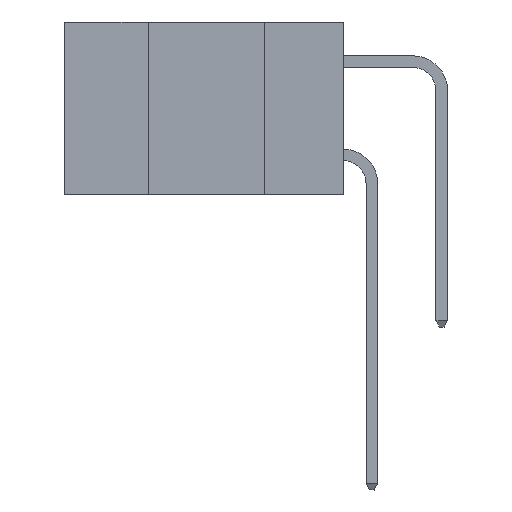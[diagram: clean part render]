
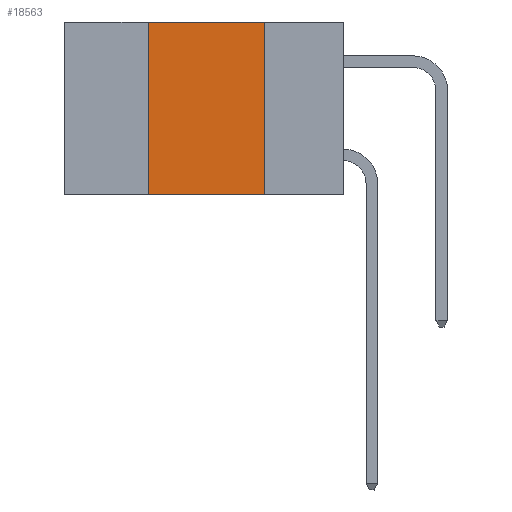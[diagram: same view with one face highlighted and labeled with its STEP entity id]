
A CAD part, left-side view. The second image highlights one B-rep face of the part: STEP entity #18563.
In plain terms, the highlighted planar face has unit normal (-1, 0, 0).
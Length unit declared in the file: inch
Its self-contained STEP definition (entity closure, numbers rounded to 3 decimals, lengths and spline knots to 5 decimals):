
#538 = CARTESIAN_POINT ( 'NONE',  ( 0., 0.42, -0.37 ) ) ;
#1553 = CARTESIAN_POINT ( 'NONE',  ( 0., 0.6, 0. ) ) ;
#1565 = VECTOR ( 'NONE', #15667, 39.37008 ) ;
#1734 = CARTESIAN_POINT ( 'NONE',  ( 0., 0.42, 0. ) ) ;
#2857 = EDGE_CURVE ( 'NONE', #12236, #12527, #21945, .T. ) ;
#3098 = PLANE ( 'NONE',  #3495 ) ;
#3495 = AXIS2_PLACEMENT_3D ( 'NONE', #11609, #20102, #5338 ) ;
#4161 = EDGE_CURVE ( 'NONE', #12236, #16341, #20436, .T. ) ;
#5338 = DIRECTION ( 'NONE',  ( 0., 0., -1. ) ) ;
#5817 = CARTESIAN_POINT ( 'NONE',  ( 0., 0.17, 0. ) ) ;
#6176 = VECTOR ( 'NONE', #16525, 39.37008 ) ;
#9912 = VERTEX_POINT ( 'NONE', #5817 ) ;
#11609 = CARTESIAN_POINT ( 'NONE',  ( 0., 0.6, 0. ) ) ;
#11755 = EDGE_LOOP ( 'NONE', ( #21059, #25407, #21462, #27111 ) ) ;
#12236 = VERTEX_POINT ( 'NONE', #538 ) ;
#12527 = VERTEX_POINT ( 'NONE', #23983 ) ;
#13703 = FACE_OUTER_BOUND ( 'NONE', #11755, .T. ) ;
#15221 = VECTOR ( 'NONE', #20825, 39.37008 ) ;
#15667 = DIRECTION ( 'NONE',  ( 0., -1., 0. ) ) ;
#16341 = VERTEX_POINT ( 'NONE', #1734 ) ;
#16525 = DIRECTION ( 'NONE',  ( 0., 0., 1. ) ) ;
#18563 = ADVANCED_FACE ( 'NONE', ( #13703 ), #3098, .F. ) ;
#19992 = CARTESIAN_POINT ( 'NONE',  ( 0., 0.6, -0.37 ) ) ;
#20102 = DIRECTION ( 'NONE',  ( 1., 0., 0. ) ) ;
#20436 = LINE ( 'NONE', #24927, #6176 ) ;
#20825 = DIRECTION ( 'NONE',  ( 0., -1., 0. ) ) ;
#20958 = LINE ( 'NONE', #1553, #15221 ) ;
#21059 = ORIENTED_EDGE ( 'NONE', *, *, #27185, .F. ) ;
#21462 = ORIENTED_EDGE ( 'NONE', *, *, #4161, .F. ) ;
#21808 = CARTESIAN_POINT ( 'NONE',  ( 0., 0.17, -0.37 ) ) ;
#21945 = LINE ( 'NONE', #19992, #1565 ) ;
#23983 = CARTESIAN_POINT ( 'NONE',  ( 0., 0.17, -0.37 ) ) ;
#24339 = LINE ( 'NONE', #21808, #25890 ) ;
#24812 = EDGE_CURVE ( 'NONE', #16341, #9912, #20958, .T. ) ;
#24927 = CARTESIAN_POINT ( 'NONE',  ( 0., 0.42, -0.37 ) ) ;
#25407 = ORIENTED_EDGE ( 'NONE', *, *, #24812, .F. ) ;
#25890 = VECTOR ( 'NONE', #26161, 39.37008 ) ;
#26161 = DIRECTION ( 'NONE',  ( 0., 0., -1. ) ) ;
#27111 = ORIENTED_EDGE ( 'NONE', *, *, #2857, .T. ) ;
#27185 = EDGE_CURVE ( 'NONE', #9912, #12527, #24339, .T. ) ;
